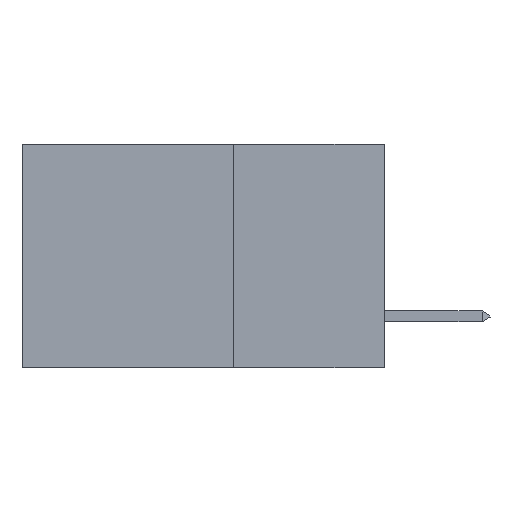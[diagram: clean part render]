
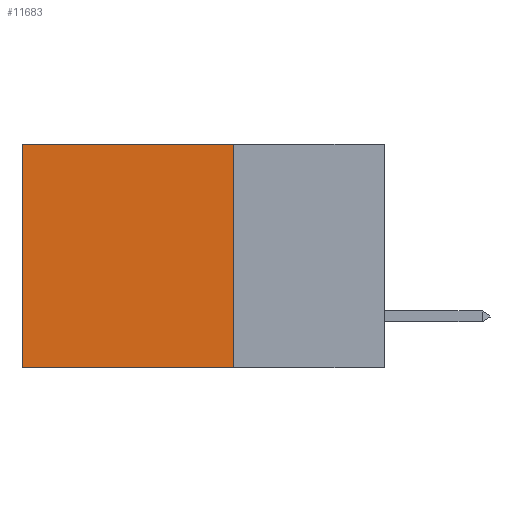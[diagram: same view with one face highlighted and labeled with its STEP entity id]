
A CAD part, left-side view. The second image highlights one B-rep face of the part: STEP entity #11683.
In plain terms, the highlighted planar face has unit normal (-1, 0, 0).
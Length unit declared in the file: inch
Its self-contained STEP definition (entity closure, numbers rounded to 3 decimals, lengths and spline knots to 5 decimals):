
#1386 = EDGE_CURVE ( 'NONE', #6252, #11552, #6533, .T. ) ;
#2175 = VECTOR ( 'NONE', #10331, 39.37008 ) ;
#2432 = EDGE_CURVE ( 'NONE', #6252, #3586, #3169, .T. ) ;
#2957 = ORIENTED_EDGE ( 'NONE', *, *, #8415, .T. ) ;
#3169 = LINE ( 'NONE', #4207, #10645 ) ;
#3586 = VERTEX_POINT ( 'NONE', #5571 ) ;
#3674 = DIRECTION ( 'NONE',  ( 1., 0., 0. ) ) ;
#4207 = CARTESIAN_POINT ( 'NONE',  ( 0.2875, 0.25, 0. ) ) ;
#4763 = ORIENTED_EDGE ( 'NONE', *, *, #2432, .T. ) ;
#4786 = PLANE ( 'NONE',  #5706 ) ;
#4834 = VERTEX_POINT ( 'NONE', #8453 ) ;
#5571 = CARTESIAN_POINT ( 'NONE',  ( 0.2875, 0.6, 0. ) ) ;
#5706 = AXIS2_PLACEMENT_3D ( 'NONE', #9777, #3674, #10799 ) ;
#6072 = VECTOR ( 'NONE', #11037, 39.37008 ) ;
#6198 = FACE_OUTER_BOUND ( 'NONE', #6402, .T. ) ;
#6252 = VERTEX_POINT ( 'NONE', #9618 ) ;
#6402 = EDGE_LOOP ( 'NONE', ( #2957, #9334, #10284, #4763 ) ) ;
#6533 = LINE ( 'NONE', #8924, #6072 ) ;
#8309 = EDGE_CURVE ( 'NONE', #11552, #4834, #9475, .T. ) ;
#8415 = EDGE_CURVE ( 'NONE', #3586, #4834, #12379, .T. ) ;
#8453 = CARTESIAN_POINT ( 'NONE',  ( 0.2875, 0.6, -0.37 ) ) ;
#8464 = CARTESIAN_POINT ( 'NONE',  ( 0.2875, 0.6, 0. ) ) ;
#8722 = CARTESIAN_POINT ( 'NONE',  ( 0.2875, 0.25, -0.37 ) ) ;
#8831 = VECTOR ( 'NONE', #10502, 39.37008 ) ;
#8924 = CARTESIAN_POINT ( 'NONE',  ( 0.2875, 0.25, 0. ) ) ;
#9298 = DIRECTION ( 'NONE',  ( 0., 1., 0. ) ) ;
#9334 = ORIENTED_EDGE ( 'NONE', *, *, #8309, .F. ) ;
#9475 = LINE ( 'NONE', #12396, #2175 ) ;
#9618 = CARTESIAN_POINT ( 'NONE',  ( 0.2875, 0.25, 0. ) ) ;
#9777 = CARTESIAN_POINT ( 'NONE',  ( 0.2875, 0.25, 0. ) ) ;
#10284 = ORIENTED_EDGE ( 'NONE', *, *, #1386, .F. ) ;
#10331 = DIRECTION ( 'NONE',  ( 0., 1., 0. ) ) ;
#10502 = DIRECTION ( 'NONE',  ( 0., 0., -1. ) ) ;
#10645 = VECTOR ( 'NONE', #9298, 39.37008 ) ;
#10799 = DIRECTION ( 'NONE',  ( 0., 0., -1. ) ) ;
#11037 = DIRECTION ( 'NONE',  ( 0., 0., -1. ) ) ;
#11552 = VERTEX_POINT ( 'NONE', #8722 ) ;
#11683 = ADVANCED_FACE ( 'NONE', ( #6198 ), #4786, .F. ) ;
#12379 = LINE ( 'NONE', #8464, #8831 ) ;
#12396 = CARTESIAN_POINT ( 'NONE',  ( 0.2875, 0.25, -0.37 ) ) ;
